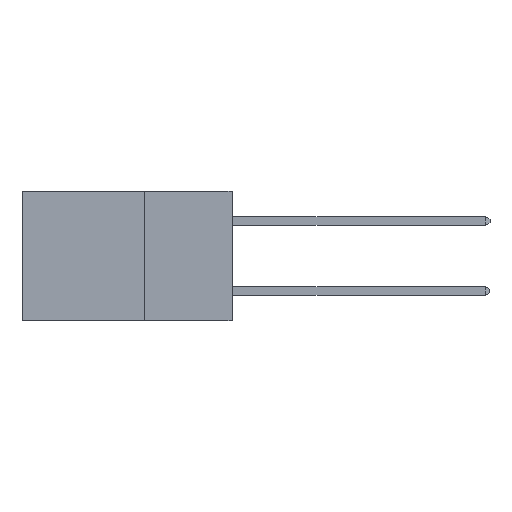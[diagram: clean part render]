
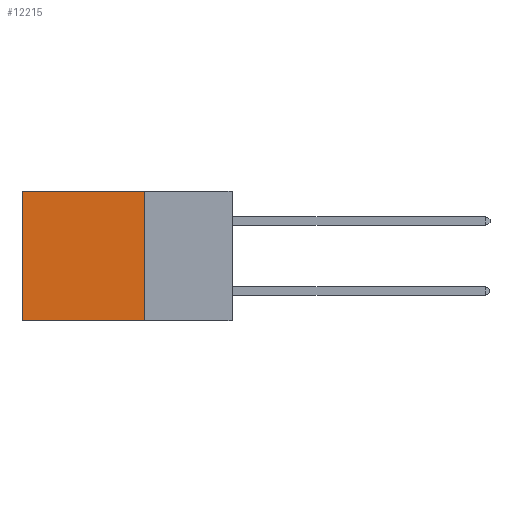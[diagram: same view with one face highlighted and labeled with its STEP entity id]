
A CAD part, left-side view. The second image highlights one B-rep face of the part: STEP entity #12215.
In plain terms, the highlighted planar face has unit normal (-1, 0, 0).
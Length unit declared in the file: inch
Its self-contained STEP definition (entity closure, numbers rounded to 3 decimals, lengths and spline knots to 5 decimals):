
#328 = LINE ( 'NONE', #8867, #8564 ) ;
#645 = EDGE_CURVE ( 'NONE', #20391, #8694, #328, .T. ) ;
#1048 = CARTESIAN_POINT ( 'NONE',  ( 0.2875, 0.25, 0. ) ) ;
#3105 = ORIENTED_EDGE ( 'NONE', *, *, #645, .T. ) ;
#3360 = CARTESIAN_POINT ( 'NONE',  ( 0.2875, 0.25, -0.37 ) ) ;
#3656 = LINE ( 'NONE', #1048, #11359 ) ;
#3703 = CARTESIAN_POINT ( 'NONE',  ( 0.2875, 0.25, 0. ) ) ;
#3864 = FACE_OUTER_BOUND ( 'NONE', #19486, .T. ) ;
#5590 = DIRECTION ( 'NONE',  ( 0., 1., 0. ) ) ;
#5804 = VECTOR ( 'NONE', #9578, 39.37008 ) ;
#6999 = DIRECTION ( 'NONE',  ( 0., 0., -1. ) ) ;
#7841 = LINE ( 'NONE', #11235, #5804 ) ;
#8564 = VECTOR ( 'NONE', #5590, 39.37008 ) ;
#8694 = VERTEX_POINT ( 'NONE', #12830 ) ;
#8867 = CARTESIAN_POINT ( 'NONE',  ( 0.2875, 0.25, 0. ) ) ;
#9255 = DIRECTION ( 'NONE',  ( 0., 0., -1. ) ) ;
#9578 = DIRECTION ( 'NONE',  ( 0., 1., 0. ) ) ;
#9900 = VERTEX_POINT ( 'NONE', #3360 ) ;
#10860 = AXIS2_PLACEMENT_3D ( 'NONE', #3703, #16766, #6999 ) ;
#11235 = CARTESIAN_POINT ( 'NONE',  ( 0.2875, 0.25, -0.37 ) ) ;
#11335 = DIRECTION ( 'NONE',  ( 0., 0., -1. ) ) ;
#11359 = VECTOR ( 'NONE', #9255, 39.37008 ) ;
#12215 = ADVANCED_FACE ( 'NONE', ( #3864 ), #13520, .F. ) ;
#12830 = CARTESIAN_POINT ( 'NONE',  ( 0.2875, 0.6, 0. ) ) ;
#13034 = ORIENTED_EDGE ( 'NONE', *, *, #21129, .F. ) ;
#13236 = VECTOR ( 'NONE', #11335, 39.37008 ) ;
#13520 = PLANE ( 'NONE',  #10860 ) ;
#13910 = ORIENTED_EDGE ( 'NONE', *, *, #18817, .T. ) ;
#15205 = EDGE_CURVE ( 'NONE', #9900, #15671, #7841, .T. ) ;
#15671 = VERTEX_POINT ( 'NONE', #17105 ) ;
#16477 = ORIENTED_EDGE ( 'NONE', *, *, #15205, .F. ) ;
#16766 = DIRECTION ( 'NONE',  ( 1., 0., 0. ) ) ;
#17105 = CARTESIAN_POINT ( 'NONE',  ( 0.2875, 0.6, -0.37 ) ) ;
#17543 = LINE ( 'NONE', #17714, #13236 ) ;
#17714 = CARTESIAN_POINT ( 'NONE',  ( 0.2875, 0.6, 0. ) ) ;
#18817 = EDGE_CURVE ( 'NONE', #8694, #15671, #17543, .T. ) ;
#19486 = EDGE_LOOP ( 'NONE', ( #13910, #16477, #13034, #3105 ) ) ;
#20391 = VERTEX_POINT ( 'NONE', #20427 ) ;
#20427 = CARTESIAN_POINT ( 'NONE',  ( 0.2875, 0.25, 0. ) ) ;
#21129 = EDGE_CURVE ( 'NONE', #20391, #9900, #3656, .T. ) ;
